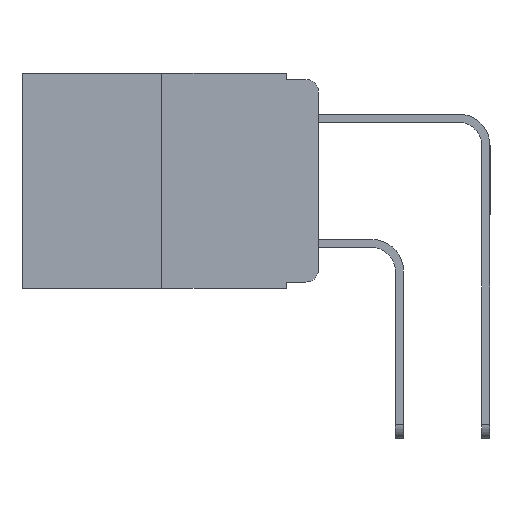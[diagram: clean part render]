
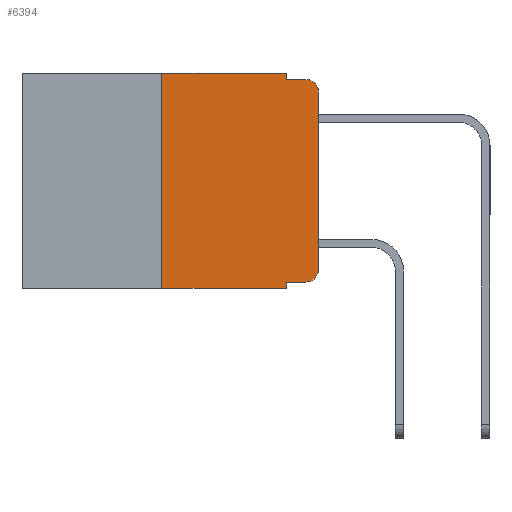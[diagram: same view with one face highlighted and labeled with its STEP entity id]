
A CAD part, left-side view. The second image highlights one B-rep face of the part: STEP entity #6394.
In plain terms, the highlighted planar face has unit normal (-1, 0, 0).
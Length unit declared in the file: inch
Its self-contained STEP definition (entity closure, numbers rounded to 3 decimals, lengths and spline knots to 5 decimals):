
#88 = VECTOR ( 'NONE', #5881, 39.37008 ) ;
#504 = CARTESIAN_POINT ( 'NONE',  ( 0., 0.25, -0.343 ) ) ;
#868 = VERTEX_POINT ( 'NONE', #8463 ) ;
#1050 = ORIENTED_EDGE ( 'NONE', *, *, #18039, .F. ) ;
#1058 = EDGE_CURVE ( 'NONE', #14372, #18099, #14032, .T. ) ;
#1420 = LINE ( 'NONE', #4938, #8986 ) ;
#1614 = VECTOR ( 'NONE', #3687, 39.37008 ) ;
#1799 = AXIS2_PLACEMENT_3D ( 'NONE', #7401, #17350, #8856 ) ;
#1886 = VERTEX_POINT ( 'NONE', #4887 ) ;
#2101 = LINE ( 'NONE', #2114, #1614 ) ;
#2102 = EDGE_CURVE ( 'NONE', #18099, #9437, #9732, .T. ) ;
#2114 = CARTESIAN_POINT ( 'NONE',  ( 0., 0.051, 0. ) ) ;
#3108 = VECTOR ( 'NONE', #5192, 39.37008 ) ;
#3133 = EDGE_CURVE ( 'NONE', #7946, #9437, #7864, .T. ) ;
#3231 = ORIENTED_EDGE ( 'NONE', *, *, #1058, .F. ) ;
#3313 = VECTOR ( 'NONE', #17126, 39.37008 ) ;
#3663 = CARTESIAN_POINT ( 'NONE',  ( 0., 0.473, -0.343 ) ) ;
#3671 = EDGE_CURVE ( 'NONE', #17384, #1886, #4230, .T. ) ;
#3687 = DIRECTION ( 'NONE',  ( 0., 0., -1. ) ) ;
#3734 = ORIENTED_EDGE ( 'NONE', *, *, #3671, .F. ) ;
#4059 = EDGE_CURVE ( 'NONE', #1886, #14372, #1420, .T. ) ;
#4099 = CARTESIAN_POINT ( 'NONE',  ( 0., 0.02, -0.01 ) ) ;
#4140 = PLANE ( 'NONE',  #6582 ) ;
#4177 = EDGE_CURVE ( 'NONE', #17227, #7946, #18468, .T. ) ;
#4230 = LINE ( 'NONE', #14596, #88 ) ;
#4668 = ORIENTED_EDGE ( 'NONE', *, *, #6851, .T. ) ;
#4887 = CARTESIAN_POINT ( 'NONE',  ( 0., 0.25, 0. ) ) ;
#4938 = CARTESIAN_POINT ( 'NONE',  ( 0., 0.473, 0. ) ) ;
#5192 = DIRECTION ( 'NONE',  ( 0., 0., 1. ) ) ;
#5881 = DIRECTION ( 'NONE',  ( 0., 0., 1. ) ) ;
#6146 = CARTESIAN_POINT ( 'NONE',  ( 0., 0.051, 0. ) ) ;
#6315 = VECTOR ( 'NONE', #8257, 39.37008 ) ;
#6353 = EDGE_LOOP ( 'NONE', ( #9796, #14058, #17740, #3231, #18572, #3734, #4668, #1050, #9570, #13838 ) ) ;
#6394 = ADVANCED_FACE ( 'NONE', ( #17024 ), #4140, .F. ) ;
#6510 = LINE ( 'NONE', #3663, #13753 ) ;
#6582 = AXIS2_PLACEMENT_3D ( 'NONE', #18461, #17152, #8652 ) ;
#6706 = CIRCLE ( 'NONE', #1799, 0.02 ) ;
#6851 = EDGE_CURVE ( 'NONE', #17384, #12956, #6510, .T. ) ;
#7359 = LINE ( 'NONE', #12930, #3313 ) ;
#7401 = CARTESIAN_POINT ( 'NONE',  ( 0., 0.02, -0.313 ) ) ;
#7864 = CIRCLE ( 'NONE', #14428, 0.02 ) ;
#7946 = VERTEX_POINT ( 'NONE', #9167 ) ;
#8076 = CARTESIAN_POINT ( 'NONE',  ( 0., 0.051, -0.343 ) ) ;
#8227 = CARTESIAN_POINT ( 'NONE',  ( 0., 0., 0. ) ) ;
#8257 = DIRECTION ( 'NONE',  ( 0., 0., -1. ) ) ;
#8463 = CARTESIAN_POINT ( 'NONE',  ( 0., 0.02, -0.333 ) ) ;
#8606 = CARTESIAN_POINT ( 'NONE',  ( 0., 0.051, 0. ) ) ;
#8652 = DIRECTION ( 'NONE',  ( 0., 0., -1. ) ) ;
#8856 = DIRECTION ( 'NONE',  ( 0., 0., -1. ) ) ;
#8986 = VECTOR ( 'NONE', #9445, 39.37008 ) ;
#9073 = CARTESIAN_POINT ( 'NONE',  ( 0., 0., -0.313 ) ) ;
#9167 = CARTESIAN_POINT ( 'NONE',  ( 0., 0., -0.03 ) ) ;
#9437 = VERTEX_POINT ( 'NONE', #4099 ) ;
#9445 = DIRECTION ( 'NONE',  ( 0., -1., 0. ) ) ;
#9570 = ORIENTED_EDGE ( 'NONE', *, *, #17123, .T. ) ;
#9732 = LINE ( 'NONE', #13846, #16375 ) ;
#9751 = CARTESIAN_POINT ( 'NONE',  ( 0., 0.051, -0.01 ) ) ;
#9796 = ORIENTED_EDGE ( 'NONE', *, *, #4177, .T. ) ;
#10709 = DIRECTION ( 'NONE',  ( 0., -1., 0. ) ) ;
#11277 = CARTESIAN_POINT ( 'NONE',  ( 0., 0.051, -0.333 ) ) ;
#11512 = VERTEX_POINT ( 'NONE', #11277 ) ;
#12930 = CARTESIAN_POINT ( 'NONE',  ( 0., 0.051, -0.333 ) ) ;
#12956 = VERTEX_POINT ( 'NONE', #8076 ) ;
#13753 = VECTOR ( 'NONE', #16705, 39.37008 ) ;
#13838 = ORIENTED_EDGE ( 'NONE', *, *, #16189, .T. ) ;
#13846 = CARTESIAN_POINT ( 'NONE',  ( 0., 0.051, -0.01 ) ) ;
#14032 = LINE ( 'NONE', #6146, #6315 ) ;
#14058 = ORIENTED_EDGE ( 'NONE', *, *, #3133, .T. ) ;
#14372 = VERTEX_POINT ( 'NONE', #8606 ) ;
#14428 = AXIS2_PLACEMENT_3D ( 'NONE', #15568, #15068, #14885 ) ;
#14596 = CARTESIAN_POINT ( 'NONE',  ( 0., 0.25, 0. ) ) ;
#14885 = DIRECTION ( 'NONE',  ( 0., 0., -1. ) ) ;
#15068 = DIRECTION ( 'NONE',  ( -1., 0., 0. ) ) ;
#15568 = CARTESIAN_POINT ( 'NONE',  ( 0., 0.02, -0.03 ) ) ;
#16189 = EDGE_CURVE ( 'NONE', #868, #17227, #6706, .T. ) ;
#16375 = VECTOR ( 'NONE', #10709, 39.37008 ) ;
#16705 = DIRECTION ( 'NONE',  ( 0., -1., 0. ) ) ;
#17024 = FACE_OUTER_BOUND ( 'NONE', #6353, .T. ) ;
#17123 = EDGE_CURVE ( 'NONE', #11512, #868, #7359, .T. ) ;
#17126 = DIRECTION ( 'NONE',  ( 0., -1., 0. ) ) ;
#17152 = DIRECTION ( 'NONE',  ( 1., 0., 0. ) ) ;
#17227 = VERTEX_POINT ( 'NONE', #9073 ) ;
#17350 = DIRECTION ( 'NONE',  ( -1., 0., 0. ) ) ;
#17384 = VERTEX_POINT ( 'NONE', #504 ) ;
#17740 = ORIENTED_EDGE ( 'NONE', *, *, #2102, .F. ) ;
#18039 = EDGE_CURVE ( 'NONE', #11512, #12956, #2101, .T. ) ;
#18099 = VERTEX_POINT ( 'NONE', #9751 ) ;
#18461 = CARTESIAN_POINT ( 'NONE',  ( 0., 0.473, 0. ) ) ;
#18468 = LINE ( 'NONE', #8227, #3108 ) ;
#18572 = ORIENTED_EDGE ( 'NONE', *, *, #4059, .F. ) ;
